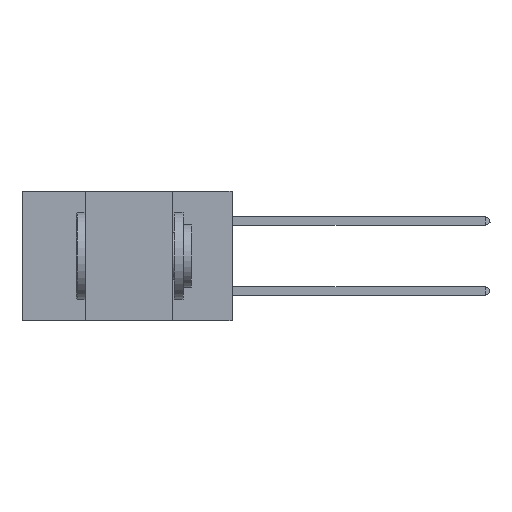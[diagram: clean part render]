
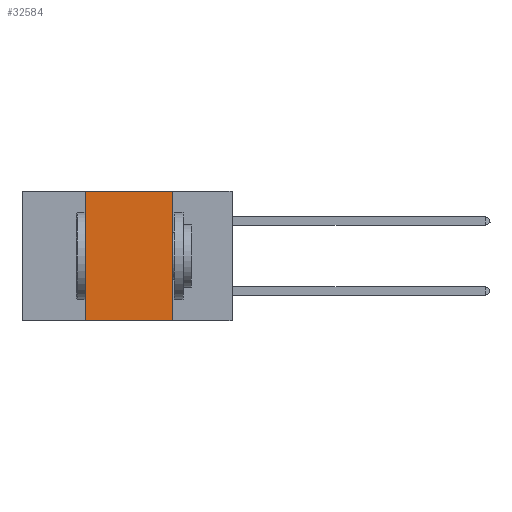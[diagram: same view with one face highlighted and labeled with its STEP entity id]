
A CAD part, left-side view. The second image highlights one B-rep face of the part: STEP entity #32584.
In plain terms, the highlighted planar face has unit normal (-1, 0, 0).
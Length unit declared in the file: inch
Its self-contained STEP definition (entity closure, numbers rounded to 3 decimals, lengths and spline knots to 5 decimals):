
#502 = DIRECTION ( 'NONE',  ( 0., 0., 1. ) ) ;
#3968 = EDGE_LOOP ( 'NONE', ( #11539, #40213, #32448, #11028 ) ) ;
#4097 = VERTEX_POINT ( 'NONE', #41093 ) ;
#6200 = FACE_OUTER_BOUND ( 'NONE', #3968, .T. ) ;
#9322 = LINE ( 'NONE', #12086, #26052 ) ;
#11028 = ORIENTED_EDGE ( 'NONE', *, *, #17071, .T. ) ;
#11369 = CARTESIAN_POINT ( 'NONE',  ( 0., 0.42, -0.37 ) ) ;
#11539 = ORIENTED_EDGE ( 'NONE', *, *, #33866, .F. ) ;
#12086 = CARTESIAN_POINT ( 'NONE',  ( 0., 0.6, 0. ) ) ;
#12623 = VECTOR ( 'NONE', #12984, 39.37008 ) ;
#12864 = DIRECTION ( 'NONE',  ( 0., -1., 0. ) ) ;
#12984 = DIRECTION ( 'NONE',  ( 0., -1., 0. ) ) ;
#13007 = CARTESIAN_POINT ( 'NONE',  ( 0., 0.17, 0. ) ) ;
#15338 = EDGE_CURVE ( 'NONE', #31567, #4097, #9322, .T. ) ;
#16065 = LINE ( 'NONE', #13007, #42594 ) ;
#17071 = EDGE_CURVE ( 'NONE', #23894, #24902, #30382, .T. ) ;
#19216 = DIRECTION ( 'NONE',  ( 1., 0., 0. ) ) ;
#23894 = VERTEX_POINT ( 'NONE', #11369 ) ;
#24313 = EDGE_CURVE ( 'NONE', #23894, #31567, #28324, .T. ) ;
#24902 = VERTEX_POINT ( 'NONE', #26655 ) ;
#26052 = VECTOR ( 'NONE', #12864, 39.37008 ) ;
#26261 = DIRECTION ( 'NONE',  ( 0., 0., -1. ) ) ;
#26655 = CARTESIAN_POINT ( 'NONE',  ( 0., 0.17, -0.37 ) ) ;
#28324 = LINE ( 'NONE', #33376, #35081 ) ;
#30382 = LINE ( 'NONE', #32960, #12623 ) ;
#31567 = VERTEX_POINT ( 'NONE', #34426 ) ;
#32448 = ORIENTED_EDGE ( 'NONE', *, *, #24313, .F. ) ;
#32584 = ADVANCED_FACE ( 'NONE', ( #6200 ), #35970, .F. ) ;
#32642 = CARTESIAN_POINT ( 'NONE',  ( 0., 0.6, 0. ) ) ;
#32960 = CARTESIAN_POINT ( 'NONE',  ( 0., 0.6, -0.37 ) ) ;
#33376 = CARTESIAN_POINT ( 'NONE',  ( 0., 0.42, 0. ) ) ;
#33866 = EDGE_CURVE ( 'NONE', #4097, #24902, #16065, .T. ) ;
#34426 = CARTESIAN_POINT ( 'NONE',  ( 0., 0.42, 0. ) ) ;
#35081 = VECTOR ( 'NONE', #502, 39.37008 ) ;
#35970 = PLANE ( 'NONE',  #39065 ) ;
#39065 = AXIS2_PLACEMENT_3D ( 'NONE', #32642, #19216, #39300 ) ;
#39300 = DIRECTION ( 'NONE',  ( 0., 0., -1. ) ) ;
#40213 = ORIENTED_EDGE ( 'NONE', *, *, #15338, .F. ) ;
#41093 = CARTESIAN_POINT ( 'NONE',  ( 0., 0.17, 0. ) ) ;
#42594 = VECTOR ( 'NONE', #26261, 39.37008 ) ;
